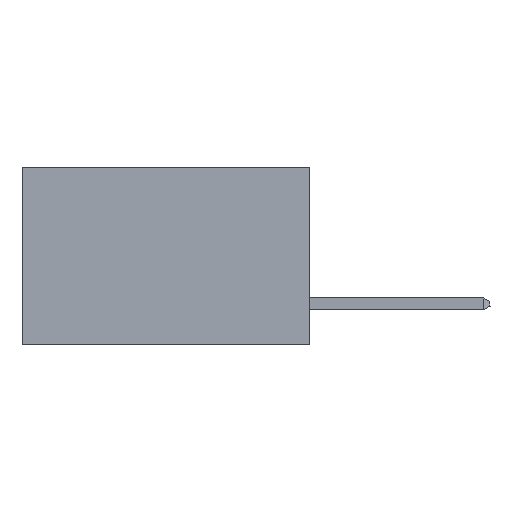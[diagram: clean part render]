
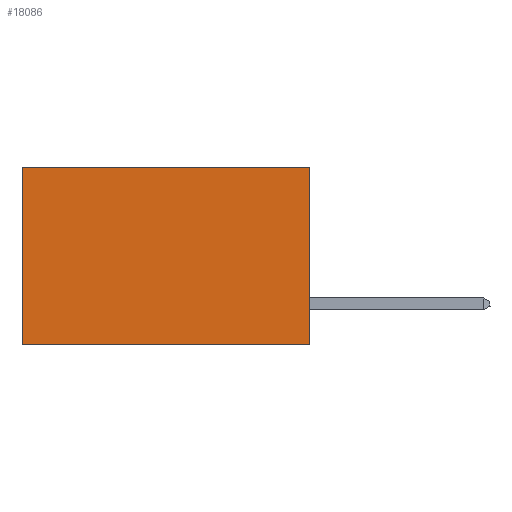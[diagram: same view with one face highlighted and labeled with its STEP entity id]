
A CAD part, left-side view. The second image highlights one B-rep face of the part: STEP entity #18086.
In plain terms, the highlighted planar face has unit normal (-1, 0, 0).
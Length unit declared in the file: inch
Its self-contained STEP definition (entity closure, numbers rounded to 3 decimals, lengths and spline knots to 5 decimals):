
#2340 = DIRECTION ( 'NONE',  ( 1., 0., 0. ) ) ;
#2437 = ORIENTED_EDGE ( 'NONE', *, *, #9694, .T. ) ;
#2867 = VERTEX_POINT ( 'NONE', #5877 ) ;
#3157 = VECTOR ( 'NONE', #15371, 39.37008 ) ;
#5087 = CARTESIAN_POINT ( 'NONE',  ( 0.2875, 0., -0.37 ) ) ;
#5877 = CARTESIAN_POINT ( 'NONE',  ( 0.2875, 0.6, -0.37 ) ) ;
#6569 = EDGE_CURVE ( 'NONE', #15413, #2867, #23167, .T. ) ;
#6901 = EDGE_CURVE ( 'NONE', #18071, #10237, #7478, .T. ) ;
#7282 = DIRECTION ( 'NONE',  ( 0., 0., -1. ) ) ;
#7478 = LINE ( 'NONE', #14233, #19169 ) ;
#8711 = EDGE_LOOP ( 'NONE', ( #2437, #9881, #10500, #15393 ) ) ;
#9694 = EDGE_CURVE ( 'NONE', #10237, #2867, #19321, .T. ) ;
#9881 = ORIENTED_EDGE ( 'NONE', *, *, #6569, .F. ) ;
#10237 = VERTEX_POINT ( 'NONE', #16231 ) ;
#10500 = ORIENTED_EDGE ( 'NONE', *, *, #18854, .F. ) ;
#11642 = PLANE ( 'NONE',  #13281 ) ;
#13150 = VECTOR ( 'NONE', #25757, 39.37008 ) ;
#13281 = AXIS2_PLACEMENT_3D ( 'NONE', #16343, #2340, #18653 ) ;
#14233 = CARTESIAN_POINT ( 'NONE',  ( 0.2875, 0., 0. ) ) ;
#15371 = DIRECTION ( 'NONE',  ( 0., 1., 0. ) ) ;
#15393 = ORIENTED_EDGE ( 'NONE', *, *, #6901, .T. ) ;
#15413 = VERTEX_POINT ( 'NONE', #5087 ) ;
#16096 = VECTOR ( 'NONE', #7282, 39.37008 ) ;
#16231 = CARTESIAN_POINT ( 'NONE',  ( 0.2875, 0.6, 0. ) ) ;
#16343 = CARTESIAN_POINT ( 'NONE',  ( 0.2875, 0., 0. ) ) ;
#18071 = VERTEX_POINT ( 'NONE', #20848 ) ;
#18086 = ADVANCED_FACE ( 'NONE', ( #20094 ), #11642, .F. ) ;
#18653 = DIRECTION ( 'NONE',  ( 0., 0., -1. ) ) ;
#18854 = EDGE_CURVE ( 'NONE', #18071, #15413, #28394, .T. ) ;
#19169 = VECTOR ( 'NONE', #28095, 39.37008 ) ;
#19321 = LINE ( 'NONE', #23390, #13150 ) ;
#20094 = FACE_OUTER_BOUND ( 'NONE', #8711, .T. ) ;
#20848 = CARTESIAN_POINT ( 'NONE',  ( 0.2875, 0., 0. ) ) ;
#23167 = LINE ( 'NONE', #26915, #3157 ) ;
#23390 = CARTESIAN_POINT ( 'NONE',  ( 0.2875, 0.6, 0. ) ) ;
#25757 = DIRECTION ( 'NONE',  ( 0., 0., -1. ) ) ;
#25847 = CARTESIAN_POINT ( 'NONE',  ( 0.2875, 0., 0. ) ) ;
#26915 = CARTESIAN_POINT ( 'NONE',  ( 0.2875, 0., -0.37 ) ) ;
#28095 = DIRECTION ( 'NONE',  ( 0., 1., 0. ) ) ;
#28394 = LINE ( 'NONE', #25847, #16096 ) ;
